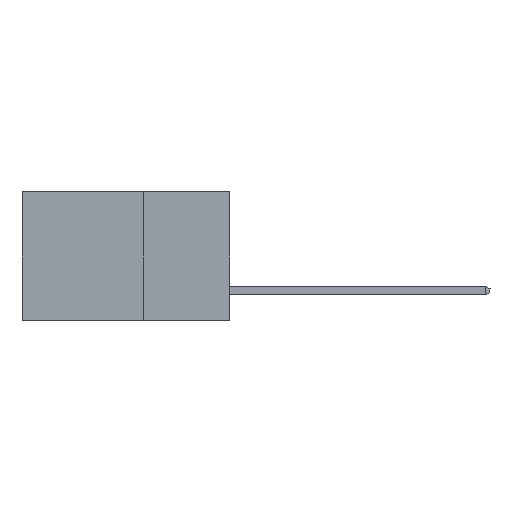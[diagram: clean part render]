
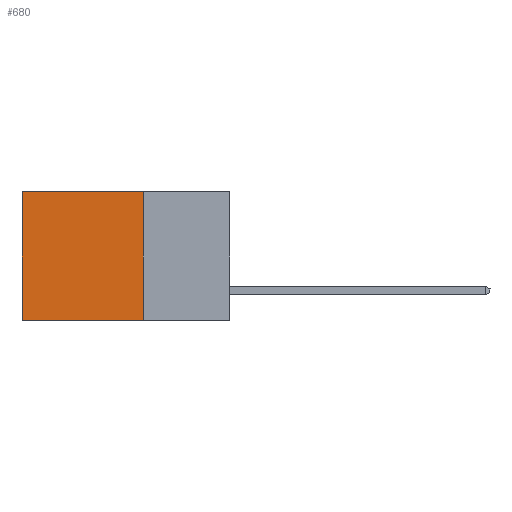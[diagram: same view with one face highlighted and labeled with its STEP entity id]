
A CAD part, left-side view. The second image highlights one B-rep face of the part: STEP entity #680.
In plain terms, the highlighted planar face has unit normal (-1, 0, 0).
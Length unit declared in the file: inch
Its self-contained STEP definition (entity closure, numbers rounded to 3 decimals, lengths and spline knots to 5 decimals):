
#680 = ADVANCED_FACE ( 'NONE', ( #17805 ), #1689, .F. ) ;
#1689 = PLANE ( 'NONE',  #18443 ) ;
#2498 = VECTOR ( 'NONE', #6502, 39.37008 ) ;
#3079 = EDGE_CURVE ( 'NONE', #18422, #10551, #7997, .T. ) ;
#3222 = VERTEX_POINT ( 'NONE', #20435 ) ;
#3428 = VECTOR ( 'NONE', #9235, 39.37008 ) ;
#3761 = LINE ( 'NONE', #11059, #3428 ) ;
#4543 = DIRECTION ( 'NONE',  ( 0., 1., 0. ) ) ;
#4579 = LINE ( 'NONE', #16914, #2498 ) ;
#4694 = DIRECTION ( 'NONE',  ( 0., 0., -1. ) ) ;
#4872 = CARTESIAN_POINT ( 'NONE',  ( 0.2615, 0.25, -0.37 ) ) ;
#6502 = DIRECTION ( 'NONE',  ( 0., 1., 0. ) ) ;
#7509 = EDGE_CURVE ( 'NONE', #18594, #3222, #3761, .T. ) ;
#7962 = CARTESIAN_POINT ( 'NONE',  ( 0.2615, 0.6, 0. ) ) ;
#7997 = LINE ( 'NONE', #13172, #20407 ) ;
#9044 = EDGE_CURVE ( 'NONE', #18422, #18594, #4579, .T. ) ;
#9235 = DIRECTION ( 'NONE',  ( 0., 0., -1. ) ) ;
#10503 = CARTESIAN_POINT ( 'NONE',  ( 0.2615, 0.25, 0. ) ) ;
#10551 = VERTEX_POINT ( 'NONE', #11183 ) ;
#10873 = ORIENTED_EDGE ( 'NONE', *, *, #15329, .F. ) ;
#10913 = ORIENTED_EDGE ( 'NONE', *, *, #3079, .F. ) ;
#11059 = CARTESIAN_POINT ( 'NONE',  ( 0.2615, 0.6, -0.37 ) ) ;
#11183 = CARTESIAN_POINT ( 'NONE',  ( 0.2615, 0.25, -0.37 ) ) ;
#13172 = CARTESIAN_POINT ( 'NONE',  ( 0.2615, 0.25, -0.37 ) ) ;
#13458 = LINE ( 'NONE', #4872, #14076 ) ;
#14076 = VECTOR ( 'NONE', #4543, 39.37008 ) ;
#14499 = EDGE_LOOP ( 'NONE', ( #19475, #10873, #10913, #17405 ) ) ;
#15329 = EDGE_CURVE ( 'NONE', #10551, #3222, #13458, .T. ) ;
#15654 = CARTESIAN_POINT ( 'NONE',  ( 0.2615, 0.25, -0.37 ) ) ;
#16328 = DIRECTION ( 'NONE',  ( 0., 0., -1. ) ) ;
#16451 = DIRECTION ( 'NONE',  ( 1., 0., 0. ) ) ;
#16914 = CARTESIAN_POINT ( 'NONE',  ( 0.2615, 0.25, 0. ) ) ;
#17405 = ORIENTED_EDGE ( 'NONE', *, *, #9044, .T. ) ;
#17805 = FACE_OUTER_BOUND ( 'NONE', #14499, .T. ) ;
#18422 = VERTEX_POINT ( 'NONE', #10503 ) ;
#18443 = AXIS2_PLACEMENT_3D ( 'NONE', #15654, #16451, #16328 ) ;
#18594 = VERTEX_POINT ( 'NONE', #7962 ) ;
#19475 = ORIENTED_EDGE ( 'NONE', *, *, #7509, .T. ) ;
#20407 = VECTOR ( 'NONE', #4694, 39.37008 ) ;
#20435 = CARTESIAN_POINT ( 'NONE',  ( 0.2615, 0.6, -0.37 ) ) ;
